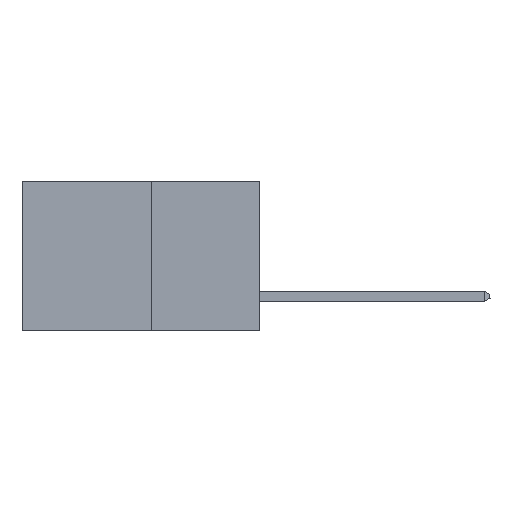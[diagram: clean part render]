
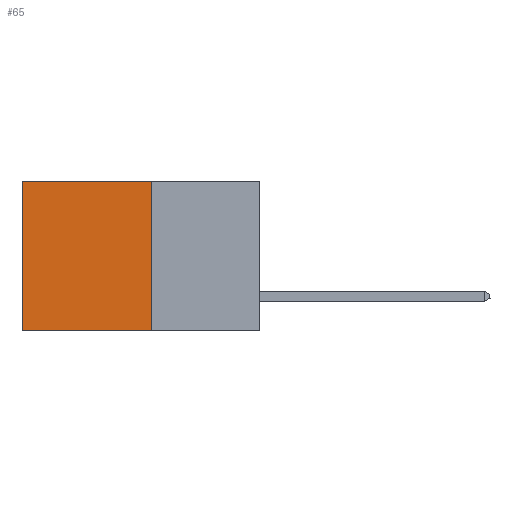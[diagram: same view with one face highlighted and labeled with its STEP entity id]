
A CAD part, left-side view. The second image highlights one B-rep face of the part: STEP entity #65.
In plain terms, the highlighted planar face has unit normal (-1, 0, 0).
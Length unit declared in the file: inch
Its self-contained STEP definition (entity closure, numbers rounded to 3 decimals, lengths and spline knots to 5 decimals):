
#65 = ADVANCED_FACE ( 'NONE', ( #5123 ), #4892, .F. ) ;
#769 = DIRECTION ( 'NONE',  ( 0., 0., -1. ) ) ;
#2024 = ORIENTED_EDGE ( 'NONE', *, *, #10645, .F. ) ;
#2517 = DIRECTION ( 'NONE',  ( 1., 0., 0. ) ) ;
#2615 = LINE ( 'NONE', #4157, #8128 ) ;
#2995 = AXIS2_PLACEMENT_3D ( 'NONE', #9814, #2517, #7061 ) ;
#3639 = VERTEX_POINT ( 'NONE', #13457 ) ;
#3926 = LINE ( 'NONE', #9049, #12215 ) ;
#4004 = VECTOR ( 'NONE', #7451, 39.37008 ) ;
#4157 = CARTESIAN_POINT ( 'NONE',  ( 0.277, 0.59, -0.37 ) ) ;
#4193 = EDGE_CURVE ( 'NONE', #9677, #3639, #12631, .T. ) ;
#4318 = EDGE_CURVE ( 'NONE', #3639, #8067, #2615, .T. ) ;
#4359 = DIRECTION ( 'NONE',  ( 0., 0., -1. ) ) ;
#4892 = PLANE ( 'NONE',  #2995 ) ;
#4989 = ORIENTED_EDGE ( 'NONE', *, *, #4193, .T. ) ;
#5123 = FACE_OUTER_BOUND ( 'NONE', #7190, .T. ) ;
#5768 = CARTESIAN_POINT ( 'NONE',  ( 0.277, 0.27, -0.37 ) ) ;
#6334 = VECTOR ( 'NONE', #769, 39.37008 ) ;
#6765 = CARTESIAN_POINT ( 'NONE',  ( 0.277, 0.59, -0.37 ) ) ;
#7061 = DIRECTION ( 'NONE',  ( 0., 0., -1. ) ) ;
#7190 = EDGE_LOOP ( 'NONE', ( #10042, #12900, #2024, #4989 ) ) ;
#7435 = CARTESIAN_POINT ( 'NONE',  ( 0.277, 0.27, 0. ) ) ;
#7451 = DIRECTION ( 'NONE',  ( 0., 1., 0. ) ) ;
#7456 = CARTESIAN_POINT ( 'NONE',  ( 0.277, 0.27, -0.37 ) ) ;
#7484 = EDGE_CURVE ( 'NONE', #11510, #8067, #3926, .T. ) ;
#8067 = VERTEX_POINT ( 'NONE', #6765 ) ;
#8128 = VECTOR ( 'NONE', #4359, 39.37008 ) ;
#8854 = LINE ( 'NONE', #7456, #6334 ) ;
#9049 = CARTESIAN_POINT ( 'NONE',  ( 0.277, 0.27, -0.37 ) ) ;
#9394 = DIRECTION ( 'NONE',  ( 0., 1., 0. ) ) ;
#9677 = VERTEX_POINT ( 'NONE', #12005 ) ;
#9814 = CARTESIAN_POINT ( 'NONE',  ( 0.277, 0.27, -0.37 ) ) ;
#10042 = ORIENTED_EDGE ( 'NONE', *, *, #4318, .T. ) ;
#10645 = EDGE_CURVE ( 'NONE', #9677, #11510, #8854, .T. ) ;
#11510 = VERTEX_POINT ( 'NONE', #5768 ) ;
#12005 = CARTESIAN_POINT ( 'NONE',  ( 0.277, 0.27, 0. ) ) ;
#12215 = VECTOR ( 'NONE', #9394, 39.37008 ) ;
#12631 = LINE ( 'NONE', #7435, #4004 ) ;
#12900 = ORIENTED_EDGE ( 'NONE', *, *, #7484, .F. ) ;
#13457 = CARTESIAN_POINT ( 'NONE',  ( 0.277, 0.59, 0. ) ) ;
